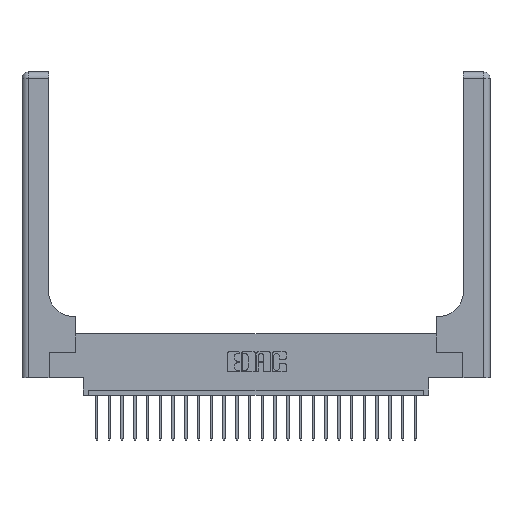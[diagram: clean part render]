
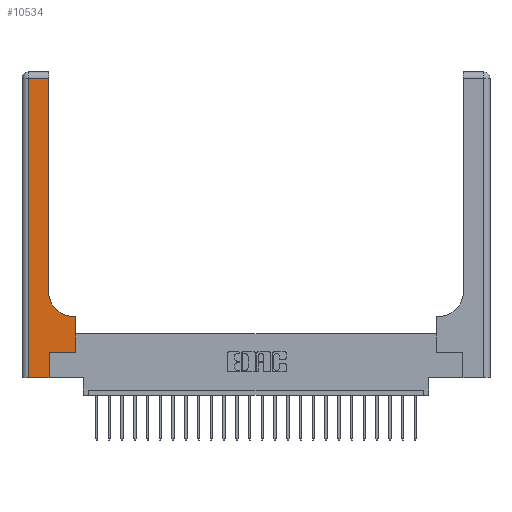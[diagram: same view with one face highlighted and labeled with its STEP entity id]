
A CAD part, top view. The second image highlights one B-rep face of the part: STEP entity #10534.
In plain terms, the highlighted planar face has unit normal (0, 0, 1).
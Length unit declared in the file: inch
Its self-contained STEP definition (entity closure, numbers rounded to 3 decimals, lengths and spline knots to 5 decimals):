
#217 = CARTESIAN_POINT ( 'NONE',  ( 0.26, 0.85, 0.37 ) ) ;
#621 = EDGE_CURVE ( 'NONE', #16195, #6357, #19353, .T. ) ;
#1182 = LINE ( 'NONE', #8607, #22438 ) ;
#1206 = EDGE_CURVE ( 'NONE', #21645, #18980, #1182, .T. ) ;
#1298 = DIRECTION ( 'NONE',  ( 0., 0., -1. ) ) ;
#1423 = DIRECTION ( 'NONE',  ( 1., 0., 0. ) ) ;
#1463 = ORIENTED_EDGE ( 'NONE', *, *, #5299, .T. ) ;
#1555 = CARTESIAN_POINT ( 'NONE',  ( 0., 3., 0.37 ) ) ;
#1972 = DIRECTION ( 'NONE',  ( 1., 0., 0. ) ) ;
#2111 = CARTESIAN_POINT ( 'NONE',  ( 0.06, 3., 0.37 ) ) ;
#2690 = EDGE_CURVE ( 'NONE', #10712, #17804, #7571, .T. ) ;
#2947 = VECTOR ( 'NONE', #9978, 39.37008 ) ;
#3334 = EDGE_LOOP ( 'NONE', ( #11697, #4032, #11872, #11966, #13361, #18390, #12774, #7219, #1463 ) ) ;
#4032 = ORIENTED_EDGE ( 'NONE', *, *, #23467, .T. ) ;
#4043 = DIRECTION ( 'NONE',  ( 0., 1., 0. ) ) ;
#4320 = LINE ( 'NONE', #15499, #7858 ) ;
#4332 = DIRECTION ( 'NONE',  ( -1., 0., 0. ) ) ;
#4972 = PLANE ( 'NONE',  #18448 ) ;
#5238 = EDGE_CURVE ( 'NONE', #9228, #15558, #4320, .T. ) ;
#5299 = EDGE_CURVE ( 'NONE', #15558, #10712, #21063, .T. ) ;
#5366 = VERTEX_POINT ( 'NONE', #6112 ) ;
#6112 = CARTESIAN_POINT ( 'NONE',  ( 0.265, 0., 0.37 ) ) ;
#6145 = EDGE_CURVE ( 'NONE', #18980, #9228, #14411, .T. ) ;
#6271 = DIRECTION ( 'NONE',  ( -1., 0., 0. ) ) ;
#6357 = VERTEX_POINT ( 'NONE', #7263 ) ;
#7219 = ORIENTED_EDGE ( 'NONE', *, *, #5238, .T. ) ;
#7263 = CARTESIAN_POINT ( 'NONE',  ( 0.06, 0., 0.37 ) ) ;
#7571 = LINE ( 'NONE', #18887, #19414 ) ;
#7816 = DIRECTION ( 'NONE',  ( 0., 0., -1. ) ) ;
#7858 = VECTOR ( 'NONE', #6271, 39.37008 ) ;
#8607 = CARTESIAN_POINT ( 'NONE',  ( 0.265, 0.25, 0.37 ) ) ;
#9228 = VERTEX_POINT ( 'NONE', #12559 ) ;
#9978 = DIRECTION ( 'NONE',  ( 0., -1., 0. ) ) ;
#10444 = VECTOR ( 'NONE', #15888, 39.37008 ) ;
#10534 = ADVANCED_FACE ( 'NONE', ( #14428 ), #4972, .F. ) ;
#10547 = CARTESIAN_POINT ( 'NONE',  ( 0.51, 0.6, 0.37 ) ) ;
#10712 = VERTEX_POINT ( 'NONE', #217 ) ;
#11593 = CARTESIAN_POINT ( 'NONE',  ( 0.06, 2.94, 0.37 ) ) ;
#11697 = ORIENTED_EDGE ( 'NONE', *, *, #2690, .T. ) ;
#11833 = LINE ( 'NONE', #19166, #16640 ) ;
#11872 = ORIENTED_EDGE ( 'NONE', *, *, #621, .T. ) ;
#11966 = ORIENTED_EDGE ( 'NONE', *, *, #23526, .T. ) ;
#12559 = CARTESIAN_POINT ( 'NONE',  ( 0.528, 0.6, 0.37 ) ) ;
#12704 = CARTESIAN_POINT ( 'NONE',  ( 0.528, 0.25, 0.37 ) ) ;
#12774 = ORIENTED_EDGE ( 'NONE', *, *, #6145, .T. ) ;
#13361 = ORIENTED_EDGE ( 'NONE', *, *, #21913, .T. ) ;
#14031 = LINE ( 'NONE', #23433, #19386 ) ;
#14411 = LINE ( 'NONE', #12704, #17197 ) ;
#14428 = FACE_OUTER_BOUND ( 'NONE', #3334, .T. ) ;
#15499 = CARTESIAN_POINT ( 'NONE',  ( 0.26, 0.6, 0.37 ) ) ;
#15533 = LINE ( 'NONE', #17595, #10444 ) ;
#15558 = VERTEX_POINT ( 'NONE', #10547 ) ;
#15888 = DIRECTION ( 'NONE',  ( 0., 1., 0. ) ) ;
#16195 = VERTEX_POINT ( 'NONE', #11593 ) ;
#16272 = CARTESIAN_POINT ( 'NONE',  ( 0.265, 0.25, 0.37 ) ) ;
#16640 = VECTOR ( 'NONE', #4332, 39.37008 ) ;
#16673 = CARTESIAN_POINT ( 'NONE',  ( 0.51, 0.85, 0.37 ) ) ;
#17197 = VECTOR ( 'NONE', #23690, 39.37008 ) ;
#17595 = CARTESIAN_POINT ( 'NONE',  ( 0.265, 0., 0.37 ) ) ;
#17804 = VERTEX_POINT ( 'NONE', #22436 ) ;
#17945 = CARTESIAN_POINT ( 'NONE',  ( 0.528, 0.25, 0.37 ) ) ;
#18294 = DIRECTION ( 'NONE',  ( 1., 0., 0. ) ) ;
#18390 = ORIENTED_EDGE ( 'NONE', *, *, #1206, .T. ) ;
#18448 = AXIS2_PLACEMENT_3D ( 'NONE', #1555, #1298, #23834 ) ;
#18887 = CARTESIAN_POINT ( 'NONE',  ( 0.26, 3., 0.37 ) ) ;
#18980 = VERTEX_POINT ( 'NONE', #17945 ) ;
#19166 = CARTESIAN_POINT ( 'NONE',  ( 0., 2.94, 0.37 ) ) ;
#19353 = LINE ( 'NONE', #2111, #2947 ) ;
#19386 = VECTOR ( 'NONE', #18294, 39.37008 ) ;
#19414 = VECTOR ( 'NONE', #4043, 39.37008 ) ;
#21063 = CIRCLE ( 'NONE', #23796, 0.25 ) ;
#21645 = VERTEX_POINT ( 'NONE', #16272 ) ;
#21913 = EDGE_CURVE ( 'NONE', #5366, #21645, #15533, .T. ) ;
#22436 = CARTESIAN_POINT ( 'NONE',  ( 0.26, 2.94, 0.37 ) ) ;
#22438 = VECTOR ( 'NONE', #1423, 39.37008 ) ;
#23433 = CARTESIAN_POINT ( 'NONE',  ( 0., 0., 0.37 ) ) ;
#23467 = EDGE_CURVE ( 'NONE', #17804, #16195, #11833, .T. ) ;
#23526 = EDGE_CURVE ( 'NONE', #6357, #5366, #14031, .T. ) ;
#23690 = DIRECTION ( 'NONE',  ( 0., 1., 0. ) ) ;
#23796 = AXIS2_PLACEMENT_3D ( 'NONE', #16673, #7816, #1972 ) ;
#23834 = DIRECTION ( 'NONE',  ( -1., 0., 0. ) ) ;
